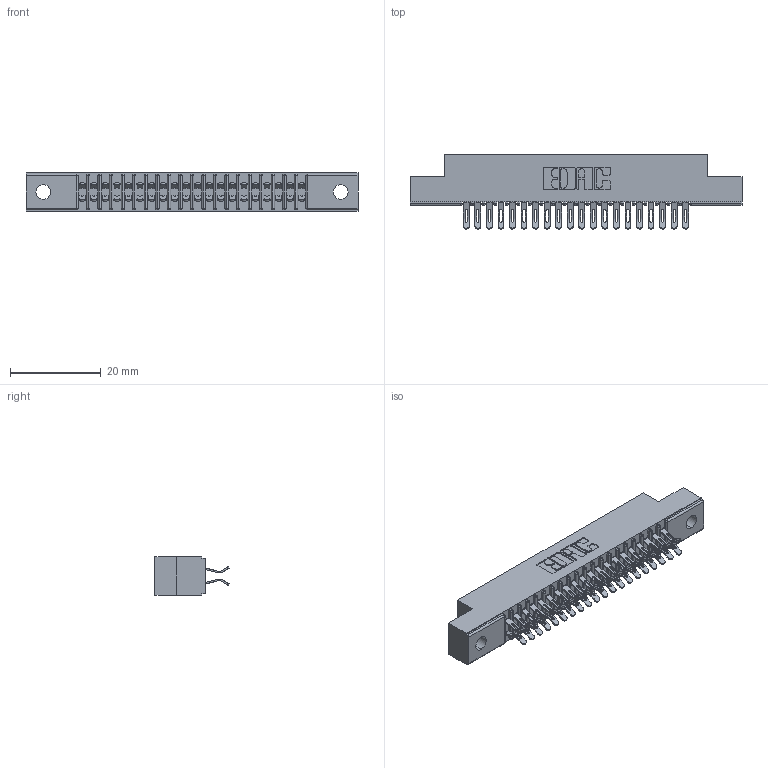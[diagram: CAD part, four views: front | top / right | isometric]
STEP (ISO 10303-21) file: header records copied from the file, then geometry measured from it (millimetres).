
FILE_DESCRIPTION (( 'STEP AP203' ), '1' );
FILE_NAME ('391-040-555-202.STEP', '2018-08-09T01:04:23', ( '' ), ( '' ), 'SwSTEP 2.0', 'SolidWorks 2016', '' );
FILE_SCHEMA (( 'CONFIG_CONTROL_DESIGN' ));
Length unit declared in the file: inch
Products named in the file (3): 341 Part_.128 (3.25) Dia Mounting Holes; 341-292-001_341-292-155; 391-040-555-202
Assembly tree (41 placements, depth 2):
  391-040-555-202
    341 Part_.128 (3.25) Dia Mounting Holes
    341-292-001_341-292-155  x40
Bounding box: 73.03 x 16.31 x 8.38 mm (x, y, z)
Volume: 4173.6 mm3; surface area: 8641.7 mm2
Topology: 41 solids, 41 shells, 3236 faces, 9656 edges, 6286 vertices
Faces by surface type: plane 1748, cylinder 1408, sphere 42, torus 38
Entity records: 27607 total; most frequent: CARTESIAN_POINT 4606, ORIENTED_EDGE 4564, DIRECTION 4476, EDGE_CURVE 2282, LINE 1804, VECTOR 1804, VERTEX_POINT 1450, AXIS2_PLACEMENT_3D 1336
